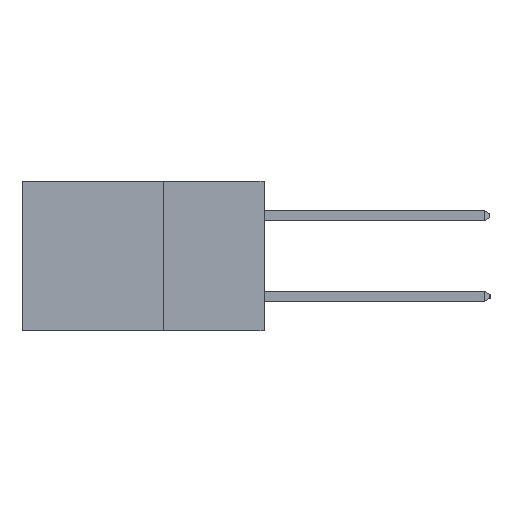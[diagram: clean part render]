
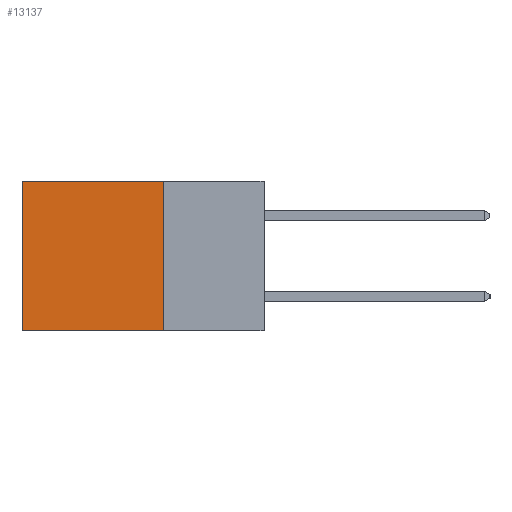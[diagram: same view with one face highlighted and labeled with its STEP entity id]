
A CAD part, left-side view. The second image highlights one B-rep face of the part: STEP entity #13137.
In plain terms, the highlighted planar face has unit normal (-1, 0, 0).
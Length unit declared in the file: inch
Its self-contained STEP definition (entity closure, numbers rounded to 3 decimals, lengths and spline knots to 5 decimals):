
#194 = DIRECTION ( 'NONE',  ( 0., 0., -1. ) ) ;
#197 = DIRECTION ( 'NONE',  ( 1., 0., 0. ) ) ;
#212 = PLANE ( 'NONE',  #7103 ) ;
#228 = CARTESIAN_POINT ( 'NONE',  ( 0.2615, 0.25, -0.37 ) ) ;
#321 = EDGE_CURVE ( 'NONE', #2381, #14701, #9383, .T. ) ;
#757 = CARTESIAN_POINT ( 'NONE',  ( 0.2615, 0.6, -0.37 ) ) ;
#1398 = ORIENTED_EDGE ( 'NONE', *, *, #2465, .T. ) ;
#1780 = VERTEX_POINT ( 'NONE', #8838 ) ;
#2381 = VERTEX_POINT ( 'NONE', #3356 ) ;
#2465 = EDGE_CURVE ( 'NONE', #8754, #14701, #2713, .T. ) ;
#2713 = LINE ( 'NONE', #11952, #15190 ) ;
#2791 = VECTOR ( 'NONE', #5699, 39.37008 ) ;
#2990 = EDGE_CURVE ( 'NONE', #1780, #8754, #15514, .T. ) ;
#3006 = DIRECTION ( 'NONE',  ( 0., 0., -1. ) ) ;
#3150 = DIRECTION ( 'NONE',  ( 0., 0., -1. ) ) ;
#3221 = CARTESIAN_POINT ( 'NONE',  ( 0.2615, 0.25, -0.37 ) ) ;
#3317 = CARTESIAN_POINT ( 'NONE',  ( 0.2615, 0.25, -0.37 ) ) ;
#3356 = CARTESIAN_POINT ( 'NONE',  ( 0.2615, 0.25, -0.37 ) ) ;
#4142 = ORIENTED_EDGE ( 'NONE', *, *, #321, .F. ) ;
#5629 = VECTOR ( 'NONE', #7288, 39.37008 ) ;
#5699 = DIRECTION ( 'NONE',  ( 0., 1., 0. ) ) ;
#7103 = AXIS2_PLACEMENT_3D ( 'NONE', #228, #197, #194 ) ;
#7288 = DIRECTION ( 'NONE',  ( 0., 1., 0. ) ) ;
#7395 = EDGE_LOOP ( 'NONE', ( #1398, #4142, #7492, #8261 ) ) ;
#7492 = ORIENTED_EDGE ( 'NONE', *, *, #9838, .F. ) ;
#8144 = VECTOR ( 'NONE', #3150, 39.37008 ) ;
#8261 = ORIENTED_EDGE ( 'NONE', *, *, #2990, .T. ) ;
#8754 = VERTEX_POINT ( 'NONE', #11047 ) ;
#8838 = CARTESIAN_POINT ( 'NONE',  ( 0.2615, 0.25, 0. ) ) ;
#9383 = LINE ( 'NONE', #3317, #2791 ) ;
#9838 = EDGE_CURVE ( 'NONE', #1780, #2381, #11708, .T. ) ;
#11047 = CARTESIAN_POINT ( 'NONE',  ( 0.2615, 0.6, 0. ) ) ;
#11708 = LINE ( 'NONE', #3221, #8144 ) ;
#11952 = CARTESIAN_POINT ( 'NONE',  ( 0.2615, 0.6, -0.37 ) ) ;
#12339 = CARTESIAN_POINT ( 'NONE',  ( 0.2615, 0.25, 0. ) ) ;
#13137 = ADVANCED_FACE ( 'NONE', ( #14162 ), #212, .F. ) ;
#14162 = FACE_OUTER_BOUND ( 'NONE', #7395, .T. ) ;
#14701 = VERTEX_POINT ( 'NONE', #757 ) ;
#15190 = VECTOR ( 'NONE', #3006, 39.37008 ) ;
#15514 = LINE ( 'NONE', #12339, #5629 ) ;
